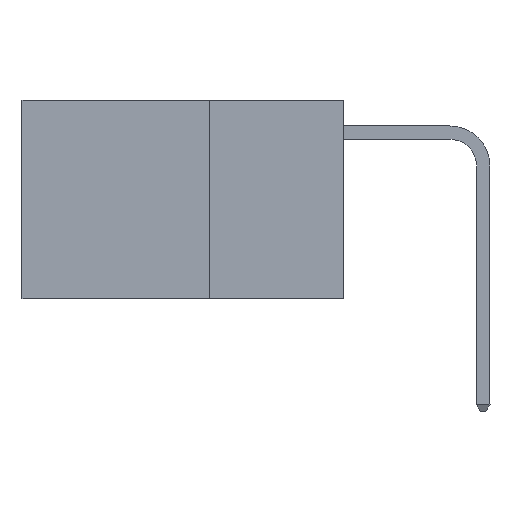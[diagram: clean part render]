
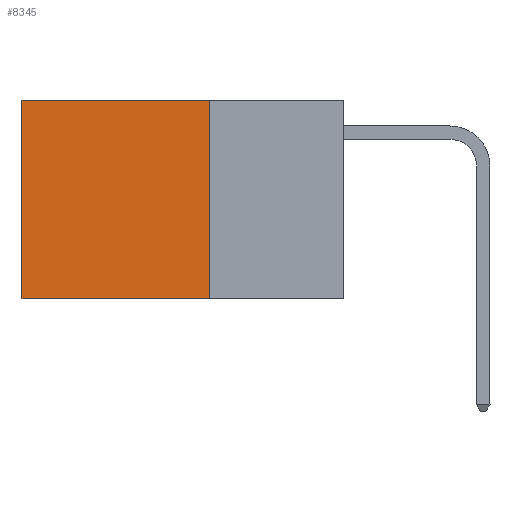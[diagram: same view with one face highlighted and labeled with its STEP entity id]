
A CAD part, left-side view. The second image highlights one B-rep face of the part: STEP entity #8345.
In plain terms, the highlighted planar face has unit normal (-1, 0, 0).
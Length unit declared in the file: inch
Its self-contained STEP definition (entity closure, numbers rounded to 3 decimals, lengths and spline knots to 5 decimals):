
#256 = EDGE_CURVE ( 'NONE', #5276, #3451, #6922, .T. ) ;
#698 = CARTESIAN_POINT ( 'NONE',  ( 0.2625, 0.6, 0. ) ) ;
#752 = PLANE ( 'NONE',  #6435 ) ;
#956 = VERTEX_POINT ( 'NONE', #2790 ) ;
#1249 = ORIENTED_EDGE ( 'NONE', *, *, #10003, .F. ) ;
#2097 = ORIENTED_EDGE ( 'NONE', *, *, #12093, .T. ) ;
#2398 = EDGE_CURVE ( 'NONE', #5276, #956, #10401, .T. ) ;
#2632 = ORIENTED_EDGE ( 'NONE', *, *, #256, .T. ) ;
#2790 = CARTESIAN_POINT ( 'NONE',  ( 0.2625, 0.25, -0.37 ) ) ;
#3105 = LINE ( 'NONE', #9460, #5424 ) ;
#3451 = VERTEX_POINT ( 'NONE', #698 ) ;
#3495 = ORIENTED_EDGE ( 'NONE', *, *, #2398, .F. ) ;
#3497 = VERTEX_POINT ( 'NONE', #11907 ) ;
#4247 = FACE_OUTER_BOUND ( 'NONE', #4677, .T. ) ;
#4609 = VECTOR ( 'NONE', #12377, 39.37008 ) ;
#4677 = EDGE_LOOP ( 'NONE', ( #2097, #1249, #3495, #2632 ) ) ;
#4881 = CARTESIAN_POINT ( 'NONE',  ( 0.2625, 0.25, 0. ) ) ;
#5223 = CARTESIAN_POINT ( 'NONE',  ( 0.2625, 0.25, 0. ) ) ;
#5227 = DIRECTION ( 'NONE',  ( 0., 0., -1. ) ) ;
#5276 = VERTEX_POINT ( 'NONE', #4881 ) ;
#5424 = VECTOR ( 'NONE', #12291, 39.37008 ) ;
#5707 = CARTESIAN_POINT ( 'NONE',  ( 0.2625, 0.25, 0. ) ) ;
#6102 = DIRECTION ( 'NONE',  ( 0., 0., -1. ) ) ;
#6435 = AXIS2_PLACEMENT_3D ( 'NONE', #5707, #12442, #6699 ) ;
#6699 = DIRECTION ( 'NONE',  ( 0., 0., -1. ) ) ;
#6922 = LINE ( 'NONE', #7432, #4609 ) ;
#7432 = CARTESIAN_POINT ( 'NONE',  ( 0.2625, 0.25, 0. ) ) ;
#7830 = VECTOR ( 'NONE', #5227, 39.37008 ) ;
#7859 = VECTOR ( 'NONE', #6102, 39.37008 ) ;
#8345 = ADVANCED_FACE ( 'NONE', ( #4247 ), #752, .F. ) ;
#9031 = CARTESIAN_POINT ( 'NONE',  ( 0.2625, 0.6, 0. ) ) ;
#9460 = CARTESIAN_POINT ( 'NONE',  ( 0.2625, 0.25, -0.37 ) ) ;
#10003 = EDGE_CURVE ( 'NONE', #956, #3497, #3105, .T. ) ;
#10401 = LINE ( 'NONE', #5223, #7830 ) ;
#10430 = LINE ( 'NONE', #9031, #7859 ) ;
#11907 = CARTESIAN_POINT ( 'NONE',  ( 0.2625, 0.6, -0.37 ) ) ;
#12093 = EDGE_CURVE ( 'NONE', #3451, #3497, #10430, .T. ) ;
#12291 = DIRECTION ( 'NONE',  ( 0., 1., 0. ) ) ;
#12377 = DIRECTION ( 'NONE',  ( 0., 1., 0. ) ) ;
#12442 = DIRECTION ( 'NONE',  ( 1., 0., 0. ) ) ;
